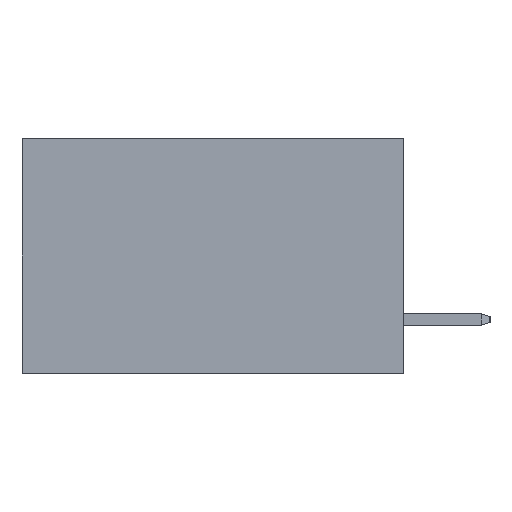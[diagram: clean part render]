
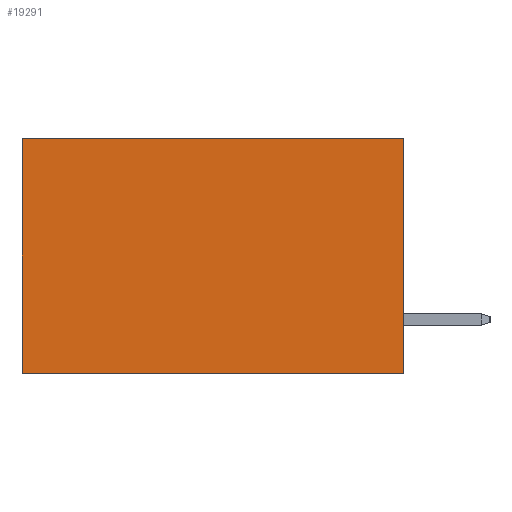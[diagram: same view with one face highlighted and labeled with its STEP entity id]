
A CAD part, left-side view. The second image highlights one B-rep face of the part: STEP entity #19291.
In plain terms, the highlighted planar face has unit normal (-1, 0, 0).
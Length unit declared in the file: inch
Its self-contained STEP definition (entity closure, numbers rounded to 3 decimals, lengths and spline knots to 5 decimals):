
#908 = CARTESIAN_POINT ( 'NONE',  ( 0.2875, 0.6, -0.37 ) ) ;
#1100 = VECTOR ( 'NONE', #7426, 39.37008 ) ;
#2335 = VERTEX_POINT ( 'NONE', #7364 ) ;
#3508 = CARTESIAN_POINT ( 'NONE',  ( 0.2875, 0.6, 0. ) ) ;
#3925 = LINE ( 'NONE', #11401, #19468 ) ;
#5062 = CARTESIAN_POINT ( 'NONE',  ( 0.2875, 0., 0. ) ) ;
#5942 = EDGE_CURVE ( 'NONE', #2335, #10349, #3925, .T. ) ;
#6484 = CARTESIAN_POINT ( 'NONE',  ( 0.2875, 0., 0. ) ) ;
#7364 = CARTESIAN_POINT ( 'NONE',  ( 0.2875, 0., -0.37 ) ) ;
#7426 = DIRECTION ( 'NONE',  ( 0., 1., 0. ) ) ;
#7600 = PLANE ( 'NONE',  #17678 ) ;
#8686 = EDGE_LOOP ( 'NONE', ( #29052, #25088, #17104, #24869 ) ) ;
#10101 = CARTESIAN_POINT ( 'NONE',  ( 0.2875, 0., 0. ) ) ;
#10136 = FACE_OUTER_BOUND ( 'NONE', #8686, .T. ) ;
#10349 = VERTEX_POINT ( 'NONE', #908 ) ;
#10837 = CARTESIAN_POINT ( 'NONE',  ( 0.2875, 0., 0. ) ) ;
#11401 = CARTESIAN_POINT ( 'NONE',  ( 0.2875, 0., -0.37 ) ) ;
#14100 = VERTEX_POINT ( 'NONE', #10837 ) ;
#15162 = LINE ( 'NONE', #3508, #23832 ) ;
#15878 = DIRECTION ( 'NONE',  ( 0., 1., 0. ) ) ;
#17104 = ORIENTED_EDGE ( 'NONE', *, *, #29523, .F. ) ;
#17678 = AXIS2_PLACEMENT_3D ( 'NONE', #5062, #23723, #28370 ) ;
#17981 = DIRECTION ( 'NONE',  ( 0., 0., -1. ) ) ;
#18536 = EDGE_CURVE ( 'NONE', #22502, #10349, #15162, .T. ) ;
#19291 = ADVANCED_FACE ( 'NONE', ( #10136 ), #7600, .F. ) ;
#19468 = VECTOR ( 'NONE', #15878, 39.37008 ) ;
#19644 = DIRECTION ( 'NONE',  ( 0., 0., -1. ) ) ;
#19833 = EDGE_CURVE ( 'NONE', #14100, #22502, #27882, .T. ) ;
#20062 = LINE ( 'NONE', #6484, #27795 ) ;
#22502 = VERTEX_POINT ( 'NONE', #22559 ) ;
#22559 = CARTESIAN_POINT ( 'NONE',  ( 0.2875, 0.6, 0. ) ) ;
#23723 = DIRECTION ( 'NONE',  ( 1., 0., 0. ) ) ;
#23832 = VECTOR ( 'NONE', #19644, 39.37008 ) ;
#24869 = ORIENTED_EDGE ( 'NONE', *, *, #19833, .T. ) ;
#25088 = ORIENTED_EDGE ( 'NONE', *, *, #5942, .F. ) ;
#27795 = VECTOR ( 'NONE', #17981, 39.37008 ) ;
#27882 = LINE ( 'NONE', #10101, #1100 ) ;
#28370 = DIRECTION ( 'NONE',  ( 0., 0., -1. ) ) ;
#29052 = ORIENTED_EDGE ( 'NONE', *, *, #18536, .T. ) ;
#29523 = EDGE_CURVE ( 'NONE', #14100, #2335, #20062, .T. ) ;
